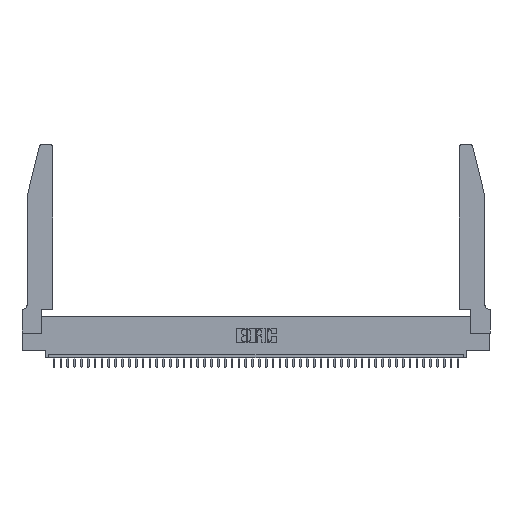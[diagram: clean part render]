
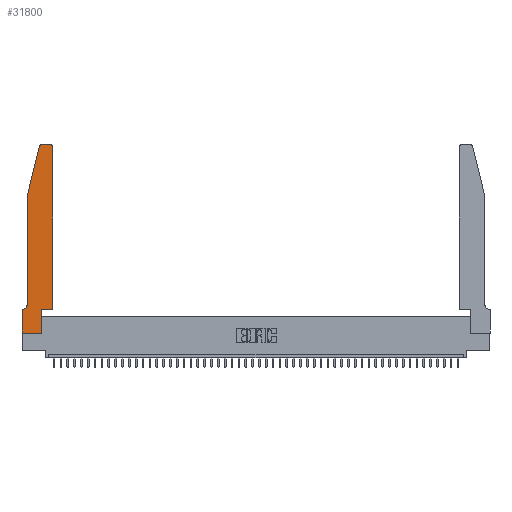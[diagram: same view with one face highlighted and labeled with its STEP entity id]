
A CAD part, top view. The second image highlights one B-rep face of the part: STEP entity #31800.
In plain terms, the highlighted planar face has unit normal (0, 0, 1).
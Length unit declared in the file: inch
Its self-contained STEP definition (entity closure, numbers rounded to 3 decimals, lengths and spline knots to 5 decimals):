
#43 = EDGE_CURVE ( 'NONE', #32572, #5843, #20616, .T. ) ;
#251 = EDGE_CURVE ( 'NONE', #47305, #37071, #14313, .T. ) ;
#410 = VERTEX_POINT ( 'NONE', #45563 ) ;
#658 = DIRECTION ( 'NONE',  ( 1., 0., 0. ) ) ;
#973 = DIRECTION ( 'NONE',  ( 1., 0., 0. ) ) ;
#1194 = CARTESIAN_POINT ( 'NONE',  ( 0.0755, 0.35, 0.37 ) ) ;
#1225 = DIRECTION ( 'NONE',  ( 0., 0., -1. ) ) ;
#1402 = CARTESIAN_POINT ( 'NONE',  ( 0., 0.35, 0.37 ) ) ;
#1602 = ORIENTED_EDGE ( 'NONE', *, *, #14951, .T. ) ;
#1608 = ORIENTED_EDGE ( 'NONE', *, *, #7606, .T. ) ;
#1922 = VERTEX_POINT ( 'NONE', #7492 ) ;
#2135 = ORIENTED_EDGE ( 'NONE', *, *, #43, .T. ) ;
#2191 = ORIENTED_EDGE ( 'NONE', *, *, #29723, .T. ) ;
#2411 = CARTESIAN_POINT ( 'NONE',  ( 0.2865, 0.35, 0.37 ) ) ;
#2733 = EDGE_CURVE ( 'NONE', #1922, #29544, #18634, .T. ) ;
#3500 = ORIENTED_EDGE ( 'NONE', *, *, #26375, .T. ) ;
#3714 = ORIENTED_EDGE ( 'NONE', *, *, #11550, .T. ) ;
#4024 = VECTOR ( 'NONE', #41277, 39.37008 ) ;
#4876 = CARTESIAN_POINT ( 'NONE',  ( 0.0755, 2., 0.37 ) ) ;
#5205 = LINE ( 'NONE', #44675, #4024 ) ;
#5269 = ORIENTED_EDGE ( 'NONE', *, *, #35659, .T. ) ;
#5283 = LINE ( 'NONE', #47640, #34000 ) ;
#5539 = VECTOR ( 'NONE', #19384, 39.37008 ) ;
#5843 = VERTEX_POINT ( 'NONE', #33743 ) ;
#6545 = VECTOR ( 'NONE', #42689, 39.37008 ) ;
#6993 = VECTOR ( 'NONE', #19686, 39.37008 ) ;
#7492 = CARTESIAN_POINT ( 'NONE',  ( 0.0755, 0.42, 0.37 ) ) ;
#7606 = EDGE_CURVE ( 'NONE', #16954, #32572, #24368, .T. ) ;
#8172 = CARTESIAN_POINT ( 'NONE',  ( 0.4505, 0.35, 0.37 ) ) ;
#8477 = CARTESIAN_POINT ( 'NONE',  ( 0.0055, 0.42, 0.37 ) ) ;
#8731 = VECTOR ( 'NONE', #658, 39.37008 ) ;
#9291 = AXIS2_PLACEMENT_3D ( 'NONE', #8477, #1225, #34141 ) ;
#9323 = CARTESIAN_POINT ( 'NONE',  ( 0.0055, 0.35, 0.37 ) ) ;
#10071 = LINE ( 'NONE', #8172, #23903 ) ;
#11130 = DIRECTION ( 'NONE',  ( 0., 0., 1. ) ) ;
#11336 = VERTEX_POINT ( 'NONE', #19200 ) ;
#11550 = EDGE_CURVE ( 'NONE', #29544, #14547, #27728, .T. ) ;
#11971 = DIRECTION ( 'NONE',  ( 0., 0., 1. ) ) ;
#12623 = DIRECTION ( 'NONE',  ( 1., 0., 0. ) ) ;
#14313 = LINE ( 'NONE', #46330, #28077 ) ;
#14547 = VERTEX_POINT ( 'NONE', #1402 ) ;
#14951 = EDGE_CURVE ( 'NONE', #37071, #1922, #47574, .T. ) ;
#14990 = DIRECTION ( 'NONE',  ( 0., 1., 0. ) ) ;
#16264 = DIRECTION ( 'NONE',  ( -1., 0., 0. ) ) ;
#16289 = CARTESIAN_POINT ( 'NONE',  ( 0.2865, 0., 0.37 ) ) ;
#16308 = ORIENTED_EDGE ( 'NONE', *, *, #251, .T. ) ;
#16954 = VERTEX_POINT ( 'NONE', #16289 ) ;
#17567 = AXIS2_PLACEMENT_3D ( 'NONE', #29790, #11971, #12623 ) ;
#18527 = CARTESIAN_POINT ( 'NONE',  ( 0.4205, 2.72, 0.37 ) ) ;
#18634 = CIRCLE ( 'NONE', #9291, 0.07 ) ;
#18669 = DIRECTION ( 'NONE',  ( 1., 0., 0. ) ) ;
#18786 = CIRCLE ( 'NONE', #40455, 0.03 ) ;
#19200 = CARTESIAN_POINT ( 'NONE',  ( 0.4505, 2.72, 0.37 ) ) ;
#19384 = DIRECTION ( 'NONE',  ( 0., -1., 0. ) ) ;
#19686 = DIRECTION ( 'NONE',  ( -1., 0., 0. ) ) ;
#20616 = LINE ( 'NONE', #33570, #33213 ) ;
#20732 = ORIENTED_EDGE ( 'NONE', *, *, #26716, .T. ) ;
#21593 = CARTESIAN_POINT ( 'NONE',  ( 0., 0., 0.37 ) ) ;
#22581 = CIRCLE ( 'NONE', #17567, 0.03 ) ;
#22716 = CARTESIAN_POINT ( 'NONE',  ( 0.284, 2.75, 0.37 ) ) ;
#22737 = ORIENTED_EDGE ( 'NONE', *, *, #2733, .T. ) ;
#23903 = VECTOR ( 'NONE', #14990, 39.37008 ) ;
#24368 = LINE ( 'NONE', #38985, #6545 ) ;
#25369 = DIRECTION ( 'NONE',  ( -0.239, -0.971, 0. ) ) ;
#25763 = EDGE_LOOP ( 'NONE', ( #20732, #3500, #16308, #1602, #22737, #3714, #5269, #29435, #1608, #2135, #2191, #38342 ) ) ;
#26375 = EDGE_CURVE ( 'NONE', #47291, #47305, #22581, .T. ) ;
#26716 = EDGE_CURVE ( 'NONE', #410, #47291, #5283, .T. ) ;
#27230 = EDGE_CURVE ( 'NONE', #39133, #16954, #47289, .T. ) ;
#27728 = LINE ( 'NONE', #1194, #6993 ) ;
#28077 = VECTOR ( 'NONE', #25369, 39.37008 ) ;
#29435 = ORIENTED_EDGE ( 'NONE', *, *, #27230, .T. ) ;
#29544 = VERTEX_POINT ( 'NONE', #9323 ) ;
#29723 = EDGE_CURVE ( 'NONE', #5843, #11336, #10071, .T. ) ;
#29790 = CARTESIAN_POINT ( 'NONE',  ( 0.284, 2.72, 0.37 ) ) ;
#31067 = FACE_OUTER_BOUND ( 'NONE', #25763, .T. ) ;
#31800 = ADVANCED_FACE ( 'NONE', ( #31067 ), #40605, .T. ) ;
#32572 = VERTEX_POINT ( 'NONE', #2411 ) ;
#32618 = DIRECTION ( 'NONE',  ( 1., 0., 0. ) ) ;
#33213 = VECTOR ( 'NONE', #973, 39.37008 ) ;
#33570 = CARTESIAN_POINT ( 'NONE',  ( 0.4505, 0.35, 0.37 ) ) ;
#33743 = CARTESIAN_POINT ( 'NONE',  ( 0.4505, 0.35, 0.37 ) ) ;
#34000 = VECTOR ( 'NONE', #16264, 39.37008 ) ;
#34141 = DIRECTION ( 'NONE',  ( -1., 0., 0. ) ) ;
#35659 = EDGE_CURVE ( 'NONE', #14547, #39133, #5205, .T. ) ;
#36456 = DIRECTION ( 'NONE',  ( 0., 0., 1. ) ) ;
#37071 = VERTEX_POINT ( 'NONE', #43929 ) ;
#38342 = ORIENTED_EDGE ( 'NONE', *, *, #43768, .T. ) ;
#38985 = CARTESIAN_POINT ( 'NONE',  ( 0.2865, 0.35, 0.37 ) ) ;
#39133 = VERTEX_POINT ( 'NONE', #40125 ) ;
#40125 = CARTESIAN_POINT ( 'NONE',  ( 0., 0., 0.37 ) ) ;
#40455 = AXIS2_PLACEMENT_3D ( 'NONE', #18527, #11130, #18669 ) ;
#40605 = PLANE ( 'NONE',  #41352 ) ;
#41277 = DIRECTION ( 'NONE',  ( 0., -1., 0. ) ) ;
#41352 = AXIS2_PLACEMENT_3D ( 'NONE', #44292, #36456, #32618 ) ;
#41356 = CARTESIAN_POINT ( 'NONE',  ( 0.25487, 2.72718, 0.37 ) ) ;
#42689 = DIRECTION ( 'NONE',  ( 0., 1., 0. ) ) ;
#43768 = EDGE_CURVE ( 'NONE', #11336, #410, #18786, .T. ) ;
#43929 = CARTESIAN_POINT ( 'NONE',  ( 0.0755, 2., 0.37 ) ) ;
#44292 = CARTESIAN_POINT ( 'NONE',  ( 0., 0.35, 0.37 ) ) ;
#44675 = CARTESIAN_POINT ( 'NONE',  ( 0., 0., 0.37 ) ) ;
#45563 = CARTESIAN_POINT ( 'NONE',  ( 0.4205, 2.75, 0.37 ) ) ;
#46330 = CARTESIAN_POINT ( 'NONE',  ( 0.0755, 2., 0.37 ) ) ;
#47289 = LINE ( 'NONE', #21593, #8731 ) ;
#47291 = VERTEX_POINT ( 'NONE', #22716 ) ;
#47305 = VERTEX_POINT ( 'NONE', #41356 ) ;
#47574 = LINE ( 'NONE', #4876, #5539 ) ;
#47640 = CARTESIAN_POINT ( 'NONE',  ( 0.2605, 2.75, 0.37 ) ) ;
